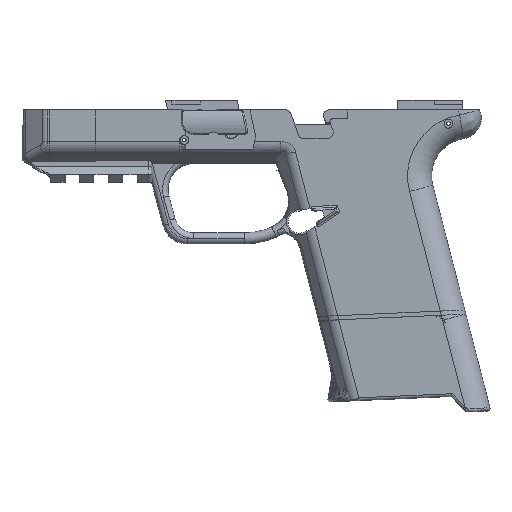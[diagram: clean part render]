
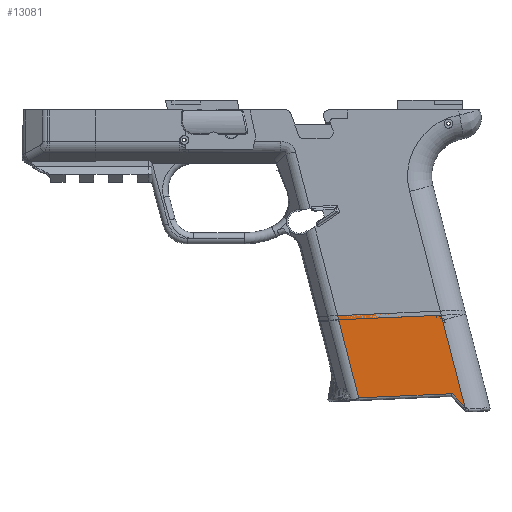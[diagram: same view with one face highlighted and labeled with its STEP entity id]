
A CAD part, left-side view. The second image highlights one B-rep face of the part: STEP entity #13081.
In plain terms, the highlighted face is planar.
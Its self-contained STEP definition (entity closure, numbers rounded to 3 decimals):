
#1064=PLANE('',#14319);
#1767=FACE_OUTER_BOUND('',#2521,.T.);
#2521=EDGE_LOOP('',(#12055,#12056,#12057,#12058,#12059));
#3636=LINE('',#25095,#4795);
#3656=LINE('',#25941,#4815);
#3670=LINE('',#26362,#4829);
#3671=LINE('',#26366,#4830);
#3672=LINE('',#26367,#4831);
#4795=VECTOR('',#17536,10.);
#4815=VECTOR('',#17628,10.);
#4829=VECTOR('',#17700,10.);
#4830=VECTOR('',#17705,10.);
#4831=VECTOR('',#17706,10.);
#6325=VERTEX_POINT('',#25073);
#6327=VERTEX_POINT('',#25093);
#6381=VERTEX_POINT('',#25940);
#6400=VERTEX_POINT('',#26203);
#6408=VERTEX_POINT('',#26365);
#8176=EDGE_CURVE('',#6327,#6325,#3636,.T.);
#8258=EDGE_CURVE('',#6381,#6325,#3656,.T.);
#8303=EDGE_CURVE('',#6400,#6327,#3670,.T.);
#8304=EDGE_CURVE('',#6408,#6400,#3671,.T.);
#8305=EDGE_CURVE('',#6408,#6381,#3672,.T.);
#12055=ORIENTED_EDGE('',*,*,#8176,.F.);
#12056=ORIENTED_EDGE('',*,*,#8303,.F.);
#12057=ORIENTED_EDGE('',*,*,#8304,.F.);
#12058=ORIENTED_EDGE('',*,*,#8305,.T.);
#12059=ORIENTED_EDGE('',*,*,#8258,.T.);
#13081=ADVANCED_FACE('',(#1767),#1064,.T.);
#14319=AXIS2_PLACEMENT_3D('',#26364,#17703,#17704);
#17536=DIRECTION('',(0.,0.999,0.044));
#17628=DIRECTION('',(0.,-0.249,0.969));
#17700=DIRECTION('',(0.,0.697,-0.717));
#17703=DIRECTION('center_axis',(1.,0.,0.));
#17704=DIRECTION('ref_axis',(0.,0.999,0.044));
#17705=DIRECTION('',(0.,-0.249,0.969));
#17706=DIRECTION('',(0.,0.999,0.044));
#25073=CARTESIAN_POINT('',(22.175,-44.727,96.906));
#25093=CARTESIAN_POINT('',(22.175,-78.67,95.402));
#25095=CARTESIAN_POINT('',(22.175,-44.598,96.911));
#25940=CARTESIAN_POINT('',(22.175,-37.062,67.087));
#25941=CARTESIAN_POINT('',(22.175,-37.062,67.087));
#26203=CARTESIAN_POINT('',(22.175,-83.249,100.107));
#26362=CARTESIAN_POINT('',(22.175,-73.025,89.603));
#26364=CARTESIAN_POINT('Origin',(22.175,-74.337,65.435));
#26365=CARTESIAN_POINT('',(22.175,-74.337,65.435));
#26366=CARTESIAN_POINT('',(22.175,-74.337,65.435));
#26367=CARTESIAN_POINT('',(22.175,-40.4,66.939));
